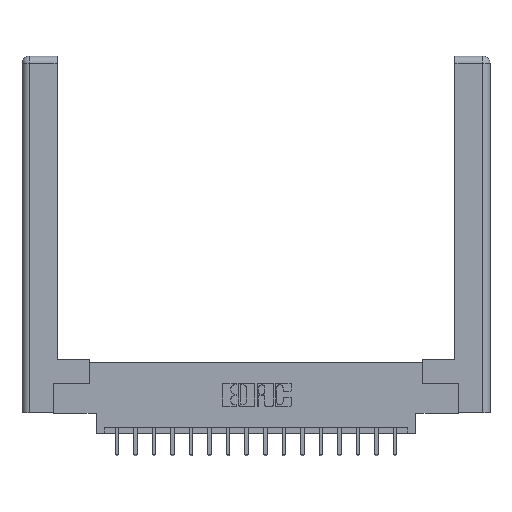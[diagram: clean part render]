
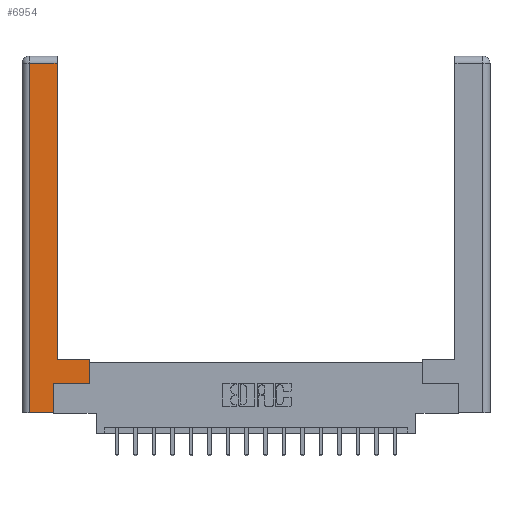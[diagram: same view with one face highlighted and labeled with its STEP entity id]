
A CAD part, top view. The second image highlights one B-rep face of the part: STEP entity #6954.
In plain terms, the highlighted planar face has unit normal (0, 0, 1).
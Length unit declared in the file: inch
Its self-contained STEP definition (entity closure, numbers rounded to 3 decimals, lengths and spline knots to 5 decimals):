
#577 = CARTESIAN_POINT ( 'NONE',  ( 0.0615, 0., 0. ) ) ;
#662 = ORIENTED_EDGE ( 'NONE', *, *, #11873, .T. ) ;
#681 = EDGE_CURVE ( 'NONE', #9159, #8697, #1119, .T. ) ;
#1119 = LINE ( 'NONE', #9545, #16048 ) ;
#1148 = DIRECTION ( 'NONE',  ( 1., 0., 0. ) ) ;
#1216 = CARTESIAN_POINT ( 'NONE',  ( 0.565, 0.245, 0. ) ) ;
#1358 = VECTOR ( 'NONE', #7571, 39.37008 ) ;
#1637 = CARTESIAN_POINT ( 'NONE',  ( 0.295, 3., 0. ) ) ;
#1875 = LINE ( 'NONE', #13220, #9286 ) ;
#2155 = DIRECTION ( 'NONE',  ( 0., -1., 0. ) ) ;
#2650 = CARTESIAN_POINT ( 'NONE',  ( 0.265, 0., 0. ) ) ;
#2867 = EDGE_LOOP ( 'NONE', ( #8400, #17298, #662, #13914, #9789, #5090, #17247, #12754 ) ) ;
#3082 = DIRECTION ( 'NONE',  ( 0., 1., 0. ) ) ;
#3313 = EDGE_CURVE ( 'NONE', #8049, #3939, #15169, .T. ) ;
#3317 = EDGE_CURVE ( 'NONE', #3939, #8307, #1875, .T. ) ;
#3939 = VERTEX_POINT ( 'NONE', #7343 ) ;
#4492 = DIRECTION ( 'NONE',  ( -1., 0., 0. ) ) ;
#4902 = CARTESIAN_POINT ( 'NONE',  ( 0.295, 0.45, 0. ) ) ;
#5090 = ORIENTED_EDGE ( 'NONE', *, *, #16601, .T. ) ;
#5162 = CARTESIAN_POINT ( 'NONE',  ( 0.565, 0.245, 0. ) ) ;
#5425 = VECTOR ( 'NONE', #3082, 39.37008 ) ;
#5779 = VERTEX_POINT ( 'NONE', #8357 ) ;
#5915 = DIRECTION ( 'NONE',  ( 0., 0., -1. ) ) ;
#6102 = PLANE ( 'NONE',  #16238 ) ;
#6290 = CARTESIAN_POINT ( 'NONE',  ( 0.265, 0.245, 0. ) ) ;
#6500 = LINE ( 'NONE', #1216, #9886 ) ;
#6639 = FACE_OUTER_BOUND ( 'NONE', #2867, .T. ) ;
#6954 = ADVANCED_FACE ( 'NONE', ( #6639 ), #6102, .F. ) ;
#7272 = DIRECTION ( 'NONE',  ( -1., 0., 0. ) ) ;
#7343 = CARTESIAN_POINT ( 'NONE',  ( 0.295, 2.94, 0. ) ) ;
#7571 = DIRECTION ( 'NONE',  ( 1., 0., 0. ) ) ;
#8049 = VERTEX_POINT ( 'NONE', #4902 ) ;
#8148 = DIRECTION ( 'NONE',  ( 0., 1., 0. ) ) ;
#8265 = VECTOR ( 'NONE', #14477, 39.37008 ) ;
#8307 = VERTEX_POINT ( 'NONE', #11810 ) ;
#8357 = CARTESIAN_POINT ( 'NONE',  ( 0.0615, 0., 0. ) ) ;
#8400 = ORIENTED_EDGE ( 'NONE', *, *, #3313, .T. ) ;
#8697 = VERTEX_POINT ( 'NONE', #6290 ) ;
#9026 = LINE ( 'NONE', #2650, #1358 ) ;
#9159 = VERTEX_POINT ( 'NONE', #14305 ) ;
#9286 = VECTOR ( 'NONE', #4492, 39.37008 ) ;
#9318 = DIRECTION ( 'NONE',  ( 0., 1., 0. ) ) ;
#9545 = CARTESIAN_POINT ( 'NONE',  ( 0.265, 0.245, 0. ) ) ;
#9789 = ORIENTED_EDGE ( 'NONE', *, *, #681, .T. ) ;
#9886 = VECTOR ( 'NONE', #1148, 39.37008 ) ;
#9933 = LINE ( 'NONE', #577, #14706 ) ;
#10143 = CARTESIAN_POINT ( 'NONE',  ( 0., 0., 0. ) ) ;
#10343 = LINE ( 'NONE', #15356, #11691 ) ;
#11691 = VECTOR ( 'NONE', #8148, 39.37008 ) ;
#11810 = CARTESIAN_POINT ( 'NONE',  ( 0.0615, 2.94, 0. ) ) ;
#11873 = EDGE_CURVE ( 'NONE', #8307, #5779, #9933, .T. ) ;
#12754 = ORIENTED_EDGE ( 'NONE', *, *, #14981, .T. ) ;
#12761 = LINE ( 'NONE', #17358, #8265 ) ;
#13220 = CARTESIAN_POINT ( 'NONE',  ( 0.0615, 2.94, 0. ) ) ;
#13603 = EDGE_CURVE ( 'NONE', #5779, #9159, #9026, .T. ) ;
#13914 = ORIENTED_EDGE ( 'NONE', *, *, #13603, .T. ) ;
#14305 = CARTESIAN_POINT ( 'NONE',  ( 0.265, 0., 0. ) ) ;
#14477 = DIRECTION ( 'NONE',  ( -1., 0., 0. ) ) ;
#14706 = VECTOR ( 'NONE', #2155, 39.37008 ) ;
#14799 = VERTEX_POINT ( 'NONE', #15820 ) ;
#14981 = EDGE_CURVE ( 'NONE', #14799, #8049, #12761, .T. ) ;
#15169 = LINE ( 'NONE', #1637, #5425 ) ;
#15356 = CARTESIAN_POINT ( 'NONE',  ( 0.565, 0.45, 0. ) ) ;
#15820 = CARTESIAN_POINT ( 'NONE',  ( 0.565, 0.45, 0. ) ) ;
#16048 = VECTOR ( 'NONE', #9318, 39.37008 ) ;
#16238 = AXIS2_PLACEMENT_3D ( 'NONE', #10143, #5915, #7272 ) ;
#16512 = EDGE_CURVE ( 'NONE', #18034, #14799, #10343, .T. ) ;
#16601 = EDGE_CURVE ( 'NONE', #8697, #18034, #6500, .T. ) ;
#17247 = ORIENTED_EDGE ( 'NONE', *, *, #16512, .T. ) ;
#17298 = ORIENTED_EDGE ( 'NONE', *, *, #3317, .T. ) ;
#17358 = CARTESIAN_POINT ( 'NONE',  ( 0.295, 0.45, 0. ) ) ;
#18034 = VERTEX_POINT ( 'NONE', #5162 ) ;
